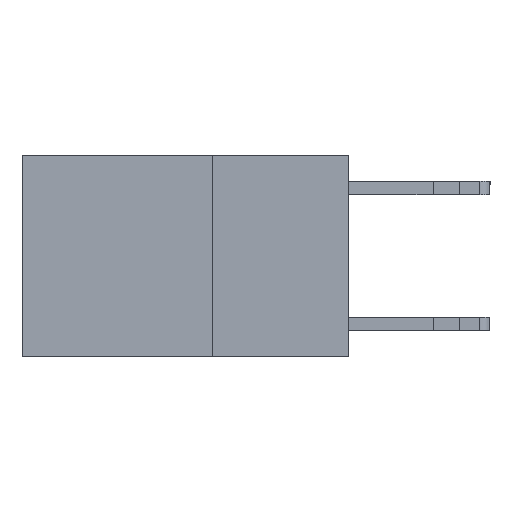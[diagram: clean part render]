
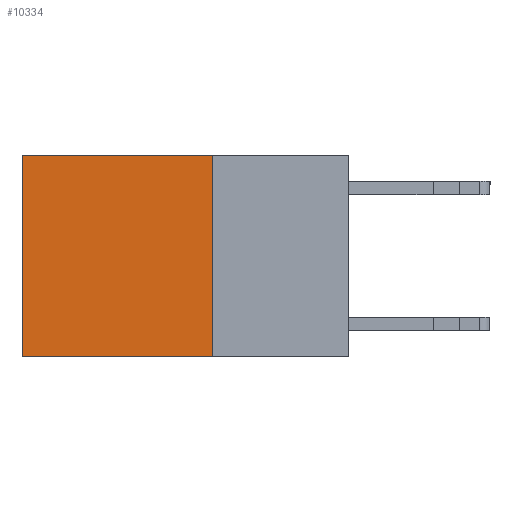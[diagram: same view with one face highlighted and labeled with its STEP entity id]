
A CAD part, left-side view. The second image highlights one B-rep face of the part: STEP entity #10334.
In plain terms, the highlighted planar face has unit normal (-1, 0, 0).
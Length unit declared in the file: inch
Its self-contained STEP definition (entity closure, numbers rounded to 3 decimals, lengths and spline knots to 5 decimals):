
#481 = ORIENTED_EDGE ( 'NONE', *, *, #1467, .F. ) ;
#1312 = CARTESIAN_POINT ( 'NONE',  ( 0.2625, 0.6, 0. ) ) ;
#1467 = EDGE_CURVE ( 'NONE', #4265, #10831, #7770, .T. ) ;
#1602 = LINE ( 'NONE', #6447, #9229 ) ;
#2067 = EDGE_CURVE ( 'NONE', #10831, #4731, #3382, .T. ) ;
#2485 = ORIENTED_EDGE ( 'NONE', *, *, #2067, .F. ) ;
#3382 = LINE ( 'NONE', #8773, #6812 ) ;
#3645 = DIRECTION ( 'NONE',  ( 1., 0., 0. ) ) ;
#4091 = VECTOR ( 'NONE', #8131, 39.37008 ) ;
#4265 = VERTEX_POINT ( 'NONE', #7487 ) ;
#4460 = DIRECTION ( 'NONE',  ( 0., 1., 0. ) ) ;
#4731 = VERTEX_POINT ( 'NONE', #10415 ) ;
#4882 = VERTEX_POINT ( 'NONE', #1312 ) ;
#5577 = AXIS2_PLACEMENT_3D ( 'NONE', #12206, #3645, #10343 ) ;
#6447 = CARTESIAN_POINT ( 'NONE',  ( 0.2625, 0.25, 0. ) ) ;
#6519 = PLANE ( 'NONE',  #5577 ) ;
#6812 = VECTOR ( 'NONE', #9766, 39.37008 ) ;
#7003 = EDGE_LOOP ( 'NONE', ( #11737, #2485, #481, #9446 ) ) ;
#7487 = CARTESIAN_POINT ( 'NONE',  ( 0.2625, 0.25, 0. ) ) ;
#7582 = DIRECTION ( 'NONE',  ( 0., 0., -1. ) ) ;
#7770 = LINE ( 'NONE', #8463, #8397 ) ;
#8131 = DIRECTION ( 'NONE',  ( 0., 0., -1. ) ) ;
#8397 = VECTOR ( 'NONE', #7582, 39.37008 ) ;
#8463 = CARTESIAN_POINT ( 'NONE',  ( 0.2625, 0.25, 0. ) ) ;
#8773 = CARTESIAN_POINT ( 'NONE',  ( 0.2625, 0.25, -0.37 ) ) ;
#9229 = VECTOR ( 'NONE', #4460, 39.37008 ) ;
#9446 = ORIENTED_EDGE ( 'NONE', *, *, #10701, .T. ) ;
#9766 = DIRECTION ( 'NONE',  ( 0., 1., 0. ) ) ;
#10136 = CARTESIAN_POINT ( 'NONE',  ( 0.2625, 0.6, 0. ) ) ;
#10195 = LINE ( 'NONE', #10136, #4091 ) ;
#10334 = ADVANCED_FACE ( 'NONE', ( #12087 ), #6519, .F. ) ;
#10343 = DIRECTION ( 'NONE',  ( 0., 0., -1. ) ) ;
#10415 = CARTESIAN_POINT ( 'NONE',  ( 0.2625, 0.6, -0.37 ) ) ;
#10560 = CARTESIAN_POINT ( 'NONE',  ( 0.2625, 0.25, -0.37 ) ) ;
#10701 = EDGE_CURVE ( 'NONE', #4265, #4882, #1602, .T. ) ;
#10831 = VERTEX_POINT ( 'NONE', #10560 ) ;
#11737 = ORIENTED_EDGE ( 'NONE', *, *, #11946, .T. ) ;
#11946 = EDGE_CURVE ( 'NONE', #4882, #4731, #10195, .T. ) ;
#12087 = FACE_OUTER_BOUND ( 'NONE', #7003, .T. ) ;
#12206 = CARTESIAN_POINT ( 'NONE',  ( 0.2625, 0.25, 0. ) ) ;
